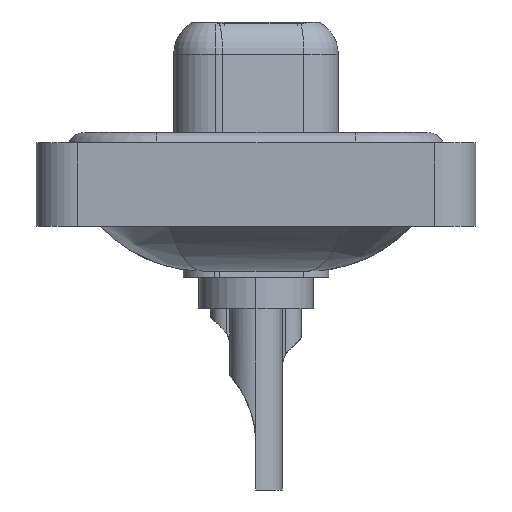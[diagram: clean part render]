
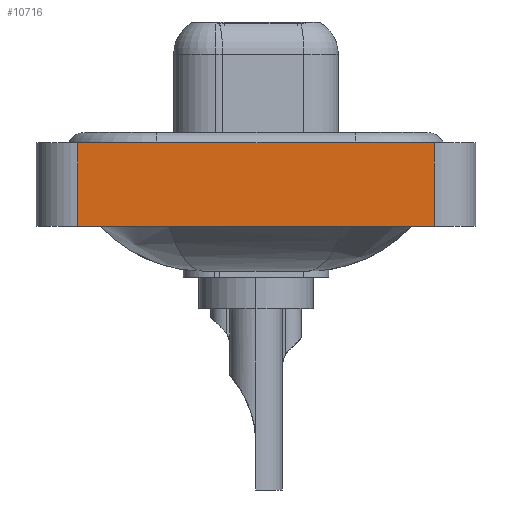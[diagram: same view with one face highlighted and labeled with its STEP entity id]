
A CAD part, left-side view. The second image highlights one B-rep face of the part: STEP entity #10716.
In plain terms, the highlighted planar face has unit normal (-1, 0, 0).
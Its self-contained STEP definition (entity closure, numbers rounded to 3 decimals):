
#1150 = CARTESIAN_POINT ( 'NONE',  ( -7.3, -8.55, -3.6 ) ) ;
#1199 = EDGE_CURVE ( 'NONE', #6701, #19377, #3959, .T. ) ;
#2465 = DIRECTION ( 'NONE',  ( 0., -1., 0. ) ) ;
#3494 = DIRECTION ( 'NONE',  ( 0., 0., 1. ) ) ;
#3577 = CARTESIAN_POINT ( 'NONE',  ( -7.3, 8.55, -3.6 ) ) ;
#3590 = CARTESIAN_POINT ( 'NONE',  ( -7.3, -8.55, -3.6 ) ) ;
#3804 = FACE_OUTER_BOUND ( 'NONE', #7552, .T. ) ;
#3823 = LINE ( 'NONE', #13187, #13523 ) ;
#3959 = LINE ( 'NONE', #1150, #6311 ) ;
#4920 = EDGE_CURVE ( 'NONE', #6994, #6701, #3823, .T. ) ;
#5088 = VERTEX_POINT ( 'NONE', #15169 ) ;
#5177 = DIRECTION ( 'NONE',  ( 0., -1., 0. ) ) ;
#5670 = LINE ( 'NONE', #5961, #12026 ) ;
#5961 = CARTESIAN_POINT ( 'NONE',  ( -7.3, -8.55, 0.4 ) ) ;
#6311 = VECTOR ( 'NONE', #7472, 1000. ) ;
#6701 = VERTEX_POINT ( 'NONE', #8100 ) ;
#6813 = PLANE ( 'NONE',  #12608 ) ;
#6994 = VERTEX_POINT ( 'NONE', #7372 ) ;
#7327 = ORIENTED_EDGE ( 'NONE', *, *, #1199, .T. ) ;
#7372 = CARTESIAN_POINT ( 'NONE',  ( -7.3, 8.55, -3.6 ) ) ;
#7472 = DIRECTION ( 'NONE',  ( 0., 0., 1. ) ) ;
#7552 = EDGE_LOOP ( 'NONE', ( #7327, #16367, #14745, #17938 ) ) ;
#8100 = CARTESIAN_POINT ( 'NONE',  ( -7.3, -8.55, -3.6 ) ) ;
#8534 = LINE ( 'NONE', #3577, #10378 ) ;
#10378 = VECTOR ( 'NONE', #16205, 1000. ) ;
#10716 = ADVANCED_FACE ( 'NONE', ( #3804 ), #6813, .T. ) ;
#11582 = DIRECTION ( 'NONE',  ( -1., 0., 0. ) ) ;
#12026 = VECTOR ( 'NONE', #2465, 1000. ) ;
#12608 = AXIS2_PLACEMENT_3D ( 'NONE', #3590, #11582, #3494 ) ;
#13187 = CARTESIAN_POINT ( 'NONE',  ( -7.3, -8.55, -3.6 ) ) ;
#13523 = VECTOR ( 'NONE', #5177, 1000. ) ;
#14745 = ORIENTED_EDGE ( 'NONE', *, *, #19898, .F. ) ;
#15169 = CARTESIAN_POINT ( 'NONE',  ( -7.3, 8.55, 0.4 ) ) ;
#16205 = DIRECTION ( 'NONE',  ( 0., 0., 1. ) ) ;
#16367 = ORIENTED_EDGE ( 'NONE', *, *, #19726, .F. ) ;
#17691 = CARTESIAN_POINT ( 'NONE',  ( -7.3, -8.55, 0.4 ) ) ;
#17938 = ORIENTED_EDGE ( 'NONE', *, *, #4920, .T. ) ;
#19377 = VERTEX_POINT ( 'NONE', #17691 ) ;
#19726 = EDGE_CURVE ( 'NONE', #5088, #19377, #5670, .T. ) ;
#19898 = EDGE_CURVE ( 'NONE', #6994, #5088, #8534, .T. ) ;
